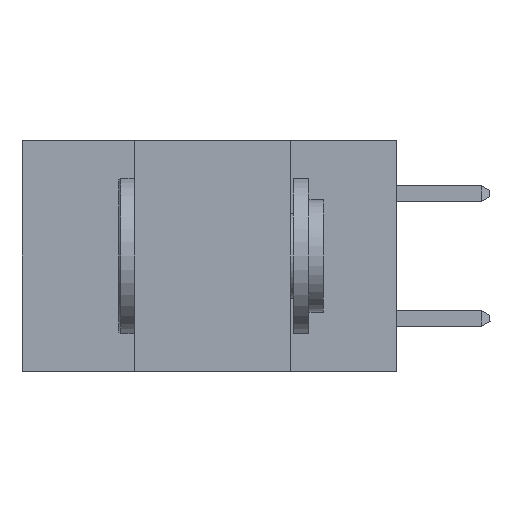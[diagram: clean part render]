
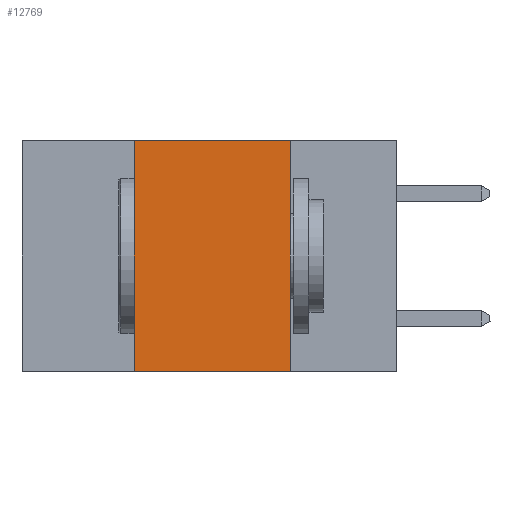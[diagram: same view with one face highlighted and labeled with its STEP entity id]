
A CAD part, left-side view. The second image highlights one B-rep face of the part: STEP entity #12769.
In plain terms, the highlighted planar face has unit normal (-1, 0, 0).
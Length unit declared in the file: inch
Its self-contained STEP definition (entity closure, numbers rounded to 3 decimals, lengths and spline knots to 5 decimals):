
#1076 = VERTEX_POINT ( 'NONE', #18917 ) ;
#2368 = VECTOR ( 'NONE', #22210, 39.37008 ) ;
#3396 = CARTESIAN_POINT ( 'NONE',  ( 0., 0.6, 0. ) ) ;
#5092 = CARTESIAN_POINT ( 'NONE',  ( 0., 0.42, 0. ) ) ;
#5170 = ORIENTED_EDGE ( 'NONE', *, *, #12426, .T. ) ;
#5543 = DIRECTION ( 'NONE',  ( 1., 0., 0. ) ) ;
#6553 = CARTESIAN_POINT ( 'NONE',  ( 0., 0.6, -0.37 ) ) ;
#6750 = LINE ( 'NONE', #5092, #17206 ) ;
#7493 = DIRECTION ( 'NONE',  ( 0., -1., 0. ) ) ;
#7797 = LINE ( 'NONE', #6553, #2368 ) ;
#8931 = VECTOR ( 'NONE', #7493, 39.37008 ) ;
#9214 = VERTEX_POINT ( 'NONE', #17075 ) ;
#9632 = EDGE_CURVE ( 'NONE', #24039, #1076, #15861, .T. ) ;
#10188 = CARTESIAN_POINT ( 'NONE',  ( 0., 0.42, -0.37 ) ) ;
#11471 = PLANE ( 'NONE',  #12425 ) ;
#12425 = AXIS2_PLACEMENT_3D ( 'NONE', #17384, #5543, #19328 ) ;
#12426 = EDGE_CURVE ( 'NONE', #24218, #1076, #7797, .T. ) ;
#12527 = DIRECTION ( 'NONE',  ( 0., 0., -1. ) ) ;
#12769 = ADVANCED_FACE ( 'NONE', ( #19399 ), #11471, .F. ) ;
#13970 = ORIENTED_EDGE ( 'NONE', *, *, #9632, .F. ) ;
#14138 = LINE ( 'NONE', #3396, #8931 ) ;
#15861 = LINE ( 'NONE', #24149, #21663 ) ;
#17075 = CARTESIAN_POINT ( 'NONE',  ( 0., 0.42, 0. ) ) ;
#17206 = VECTOR ( 'NONE', #18897, 39.37008 ) ;
#17384 = CARTESIAN_POINT ( 'NONE',  ( 0., 0.6, 0. ) ) ;
#17741 = ORIENTED_EDGE ( 'NONE', *, *, #24485, .F. ) ;
#18845 = EDGE_LOOP ( 'NONE', ( #13970, #21570, #17741, #5170 ) ) ;
#18897 = DIRECTION ( 'NONE',  ( 0., 0., 1. ) ) ;
#18917 = CARTESIAN_POINT ( 'NONE',  ( 0., 0.17, -0.37 ) ) ;
#19328 = DIRECTION ( 'NONE',  ( 0., 0., -1. ) ) ;
#19399 = FACE_OUTER_BOUND ( 'NONE', #18845, .T. ) ;
#21570 = ORIENTED_EDGE ( 'NONE', *, *, #24629, .F. ) ;
#21663 = VECTOR ( 'NONE', #12527, 39.37008 ) ;
#22210 = DIRECTION ( 'NONE',  ( 0., -1., 0. ) ) ;
#24039 = VERTEX_POINT ( 'NONE', #25245 ) ;
#24149 = CARTESIAN_POINT ( 'NONE',  ( 0., 0.17, 0. ) ) ;
#24218 = VERTEX_POINT ( 'NONE', #10188 ) ;
#24485 = EDGE_CURVE ( 'NONE', #24218, #9214, #6750, .T. ) ;
#24629 = EDGE_CURVE ( 'NONE', #9214, #24039, #14138, .T. ) ;
#25245 = CARTESIAN_POINT ( 'NONE',  ( 0., 0.17, 0. ) ) ;
